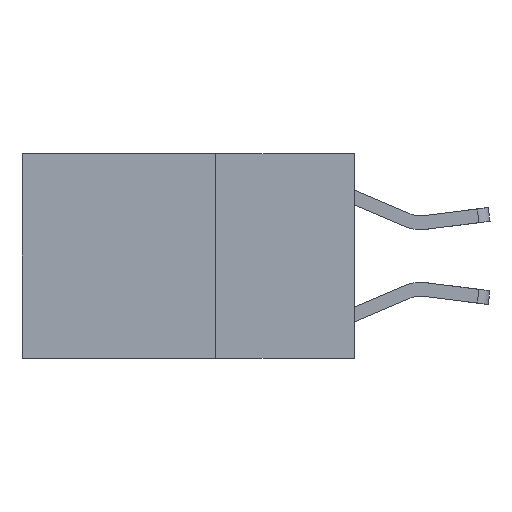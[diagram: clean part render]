
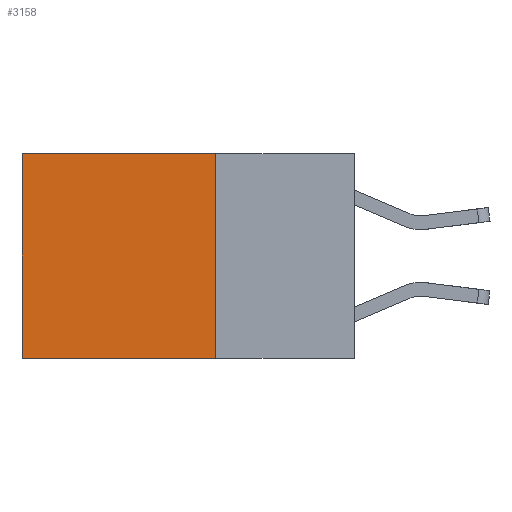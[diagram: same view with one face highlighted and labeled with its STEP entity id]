
A CAD part, left-side view. The second image highlights one B-rep face of the part: STEP entity #3158.
In plain terms, the highlighted planar face has unit normal (-1, 0, 0).
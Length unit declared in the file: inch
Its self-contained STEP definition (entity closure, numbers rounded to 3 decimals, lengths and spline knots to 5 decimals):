
#450 = EDGE_CURVE ( 'NONE', #1437, #3522, #3753, .T. ) ;
#499 = VERTEX_POINT ( 'NONE', #5912 ) ;
#1005 = VECTOR ( 'NONE', #5776, 39.37008 ) ;
#1238 = PLANE ( 'NONE',  #4881 ) ;
#1378 = VECTOR ( 'NONE', #3761, 39.37008 ) ;
#1437 = VERTEX_POINT ( 'NONE', #3812 ) ;
#1700 = CARTESIAN_POINT ( 'NONE',  ( 0.2625, 0.6, -0.37 ) ) ;
#1982 = DIRECTION ( 'NONE',  ( 1., 0., 0. ) ) ;
#2805 = LINE ( 'NONE', #3736, #1378 ) ;
#3146 = CARTESIAN_POINT ( 'NONE',  ( 0.2625, 0.25, 0. ) ) ;
#3158 = ADVANCED_FACE ( 'NONE', ( #5159 ), #1238, .F. ) ;
#3205 = VERTEX_POINT ( 'NONE', #6591 ) ;
#3463 = ORIENTED_EDGE ( 'NONE', *, *, #5664, .F. ) ;
#3491 = VECTOR ( 'NONE', #3930, 39.37008 ) ;
#3522 = VERTEX_POINT ( 'NONE', #1700 ) ;
#3736 = CARTESIAN_POINT ( 'NONE',  ( 0.2625, 0.6, 0. ) ) ;
#3753 = LINE ( 'NONE', #5630, #1005 ) ;
#3761 = DIRECTION ( 'NONE',  ( 0., 0., -1. ) ) ;
#3788 = LINE ( 'NONE', #3146, #7128 ) ;
#3812 = CARTESIAN_POINT ( 'NONE',  ( 0.2625, 0.25, -0.37 ) ) ;
#3930 = DIRECTION ( 'NONE',  ( 0., 0., -1. ) ) ;
#4106 = DIRECTION ( 'NONE',  ( 0., 0., -1. ) ) ;
#4407 = EDGE_LOOP ( 'NONE', ( #6936, #8726, #3463, #6814 ) ) ;
#4768 = CARTESIAN_POINT ( 'NONE',  ( 0.2625, 0.25, 0. ) ) ;
#4881 = AXIS2_PLACEMENT_3D ( 'NONE', #4768, #1982, #4106 ) ;
#5159 = FACE_OUTER_BOUND ( 'NONE', #4407, .T. ) ;
#5630 = CARTESIAN_POINT ( 'NONE',  ( 0.2625, 0.25, -0.37 ) ) ;
#5664 = EDGE_CURVE ( 'NONE', #499, #1437, #5691, .T. ) ;
#5691 = LINE ( 'NONE', #8112, #3491 ) ;
#5776 = DIRECTION ( 'NONE',  ( 0., 1., 0. ) ) ;
#5912 = CARTESIAN_POINT ( 'NONE',  ( 0.2625, 0.25, 0. ) ) ;
#6123 = DIRECTION ( 'NONE',  ( 0., 1., 0. ) ) ;
#6591 = CARTESIAN_POINT ( 'NONE',  ( 0.2625, 0.6, 0. ) ) ;
#6814 = ORIENTED_EDGE ( 'NONE', *, *, #8075, .T. ) ;
#6936 = ORIENTED_EDGE ( 'NONE', *, *, #8637, .T. ) ;
#7128 = VECTOR ( 'NONE', #6123, 39.37008 ) ;
#8075 = EDGE_CURVE ( 'NONE', #499, #3205, #3788, .T. ) ;
#8112 = CARTESIAN_POINT ( 'NONE',  ( 0.2625, 0.25, 0. ) ) ;
#8637 = EDGE_CURVE ( 'NONE', #3205, #3522, #2805, .T. ) ;
#8726 = ORIENTED_EDGE ( 'NONE', *, *, #450, .F. ) ;
